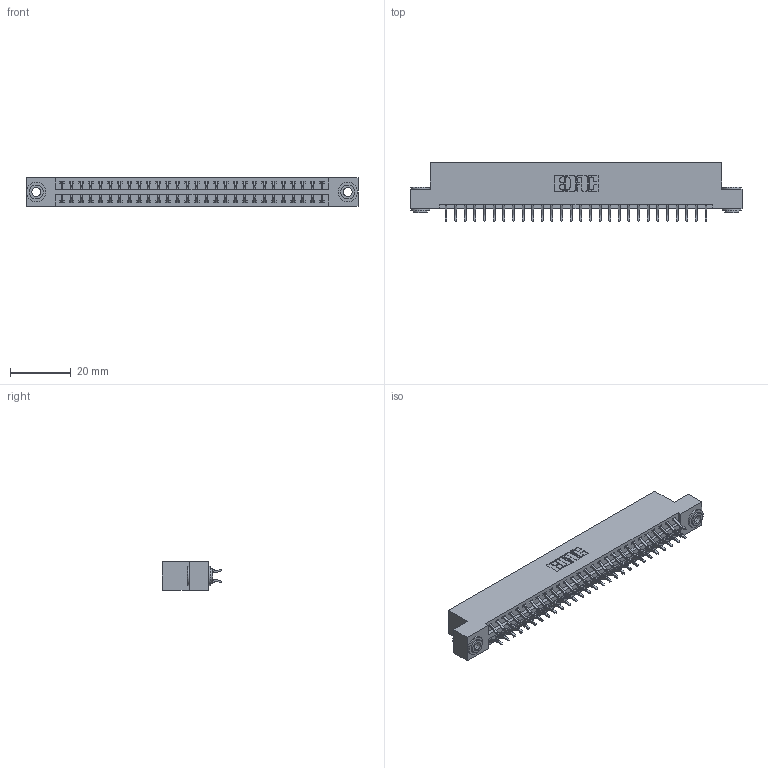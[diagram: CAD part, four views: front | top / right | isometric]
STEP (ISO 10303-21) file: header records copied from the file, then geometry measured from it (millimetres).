
FILE_DESCRIPTION (( 'STEP AP203' ), '1' );
FILE_NAME ('346-056-556-203.STEP', '2022-05-21T06:26:41', ( '' ), ( '' ), 'SwSTEP 2.0', 'SolidWorks 2020', '' );
FILE_SCHEMA (( 'CONFIG_CONTROL_DESIGN' ));
Length unit declared in the file: inch
Products named in the file (4): 346-056-556-203; 345-250-002_345-250-002-102; 345-292-001_556 Tail; 346 Part_Flush Mounting Lugs - 0.156 Dia-TH
Assembly tree (59 placements, depth 2):
  346-056-556-203
    346 Part_Flush Mounting Lugs - 0.156 Dia-TH
    345-292-001_556 Tail  x56
    345-250-002_345-250-002-102  x2
Bounding box: 109.47 x 19.57 x 9.4 mm (x, y, z)
Volume: 10565.4 mm3; surface area: 14499.5 mm2
Topology: 59 solids, 59 shells, 3422 faces, 10129 edges, 6674 vertices
Faces by surface type: plane 2284, cylinder 1130, cone 8
Entity records: 21444 total; most frequent: CARTESIAN_POINT 3549, ORIENTED_EDGE 3462, DIRECTION 3197, EDGE_CURVE 1731, VECTOR 1455, LINE 1455, VERTEX_POINT 1150, AXIS2_PLACEMENT_3D 871
